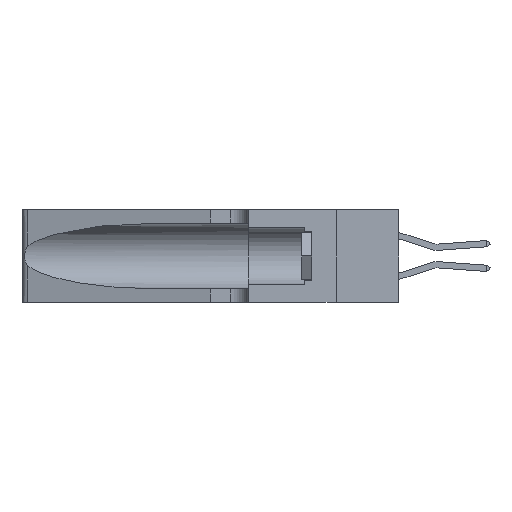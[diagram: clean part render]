
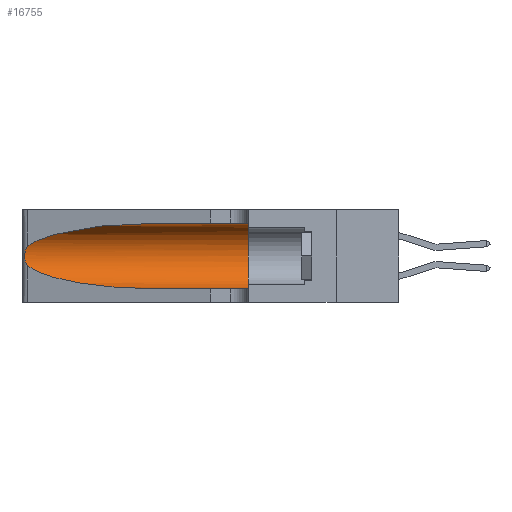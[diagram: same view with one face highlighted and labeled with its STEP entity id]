
A CAD part, left-side view. The second image highlights one B-rep face of the part: STEP entity #16755.
In plain terms, the highlighted cylindrical face has radius 3.308 mm (diameter 6.617 mm), a partial arc.
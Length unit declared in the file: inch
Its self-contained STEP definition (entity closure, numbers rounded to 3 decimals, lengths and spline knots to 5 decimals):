
#390 = VERTEX_POINT ( 'NONE', #656 ) ;
#656 = CARTESIAN_POINT ( 'NONE',  ( 0.1305, 0.35, 0.05475 ) ) ;
#829 = ORIENTED_EDGE ( 'NONE', *, *, #35304, .F. ) ;
#1144 = EDGE_CURVE ( 'NONE', #29607, #32186, #32940, .T. ) ;
#1484 = DIRECTION ( 'NONE',  ( 0., 0., -1. ) ) ;
#1635 = VERTEX_POINT ( 'NONE', #23614 ) ;
#3632 = CARTESIAN_POINT ( 'NONE',  ( 0.25555, 1.22993, 0.14849 ) ) ;
#4254 = CARTESIAN_POINT ( 'NONE',  ( 0.18966, 0.96281, 0.05475 ) ) ;
#4380 = CARTESIAN_POINT ( 'NONE',  ( 0.1305, 1.61858, 0.185 ) ) ;
#4558 = ORIENTED_EDGE ( 'NONE', *, *, #1144, .T. ) ;
#5376 = VECTOR ( 'NONE', #12789, 39.37008 ) ;
#6652 = EDGE_CURVE ( 'NONE', #27909, #29607, #11168, .T. ) ;
#6668 = ORIENTED_EDGE ( 'NONE', *, *, #27899, .T. ) ;
#6998 = CARTESIAN_POINT ( 'NONE',  ( 0.25789, 1.23486, 0.15765 ) ) ;
#7137 = CARTESIAN_POINT ( 'NONE',  ( 0.25555, 1.22994, 0.2215 ) ) ;
#7520 = FACE_OUTER_BOUND ( 'NONE', #35198, .T. ) ;
#7608 = CARTESIAN_POINT ( 'NONE',  ( 0.25487, 1.22718, 0.14631 ) ) ;
#8059 = EDGE_CURVE ( 'NONE', #1635, #27909, #25760, .T. ) ;
#9537 = CARTESIAN_POINT ( 'NONE',  ( 0.25487, 1.22718, 0.14631 ) ) ;
#10069 = CARTESIAN_POINT ( 'NONE',  ( 0.26018, 1.23835, 0.19895 ) ) ;
#11168 = B_SPLINE_CURVE_WITH_KNOTS ( 'NONE', 3,
 ( #29820, #7137, #30094, #43023, #23140, #10069, #26786, #39811, #36946, #39675, #6998, #33306, #3632, #30233 ),
 .UNSPECIFIED., .F., .F.,
 ( 4, 2, 2, 2, 2, 2, 4 ),
 ( 0., 0.00027, 0.00053, 0.00107, 0.0016, 0.00187, 0.00214 ),
 .UNSPECIFIED. ) ;
#11863 = CARTESIAN_POINT ( 'NONE',  ( 0.1305, 0.72297, 0.05475 ) ) ;
#12789 = DIRECTION ( 'NONE',  ( 0., -1., 0. ) ) ;
#14863 = CYLINDRICAL_SURFACE ( 'NONE', #21167, 0.13025 ) ;
#15998 = EDGE_CURVE ( 'NONE', #28734, #390, #23741, .T. ) ;
#16018 = CARTESIAN_POINT ( 'NONE',  ( 0.18966, 0.96281, 0.31525 ) ) ;
#16755 = ADVANCED_FACE ( 'NONE', ( #7520 ), #14863, .F. ) ;
#17876 = CARTESIAN_POINT ( 'NONE',  ( 0.1305, 0.35, 0.185 ) ) ;
#18676 = CARTESIAN_POINT ( 'NONE',  ( 0.1305, 1.61858, 0.05475 ) ) ;
#20584 = AXIS2_PLACEMENT_3D ( 'NONE', #17876, #34741, #35028 ) ;
#21167 = AXIS2_PLACEMENT_3D ( 'NONE', #4380, #34636, #1484 ) ;
#22700 = VECTOR ( 'NONE', #31290, 39.37008 ) ;
#23140 = CARTESIAN_POINT ( 'NONE',  ( 0.25854, 1.2359, 0.20912 ) ) ;
#23196 = CARTESIAN_POINT ( 'NONE',  ( 0.1305, 0.35, 0.31525 ) ) ;
#23614 = CARTESIAN_POINT ( 'NONE',  ( 0.1305, 0.72297, 0.31525 ) ) ;
#23741 = CIRCLE ( 'NONE', #20584, 0.13025 ) ;
#25760 =( BOUNDED_CURVE ( )  B_SPLINE_CURVE ( 3, ( #32696, #16018, #42717, #32416 ),
 .UNSPECIFIED., .F., .F. ) 
 B_SPLINE_CURVE_WITH_KNOTS ( ( 4, 4 ),
 ( 1.5708, 2.84003 ),
 .UNSPECIFIED. ) 
 CURVE ( )  GEOMETRIC_REPRESENTATION_ITEM ( )  RATIONAL_B_SPLINE_CURVE ( ( 1., 0.87, 0.87, 1. ) ) 
 REPRESENTATION_ITEM ( '' )  );
#26551 = ORIENTED_EDGE ( 'NONE', *, *, #6652, .T. ) ;
#26786 = CARTESIAN_POINT ( 'NONE',  ( 0.26075, 1.23896, 0.19203 ) ) ;
#27537 = CARTESIAN_POINT ( 'NONE',  ( 0.1305, 0.72297, 0.05475 ) ) ;
#27759 = ORIENTED_EDGE ( 'NONE', *, *, #15998, .F. ) ;
#27899 = EDGE_CURVE ( 'NONE', #32186, #390, #40351, .T. ) ;
#27909 = VERTEX_POINT ( 'NONE', #42315 ) ;
#28666 = ORIENTED_EDGE ( 'NONE', *, *, #8059, .T. ) ;
#28734 = VERTEX_POINT ( 'NONE', #23196 ) ;
#29607 = VERTEX_POINT ( 'NONE', #9537 ) ;
#29820 = CARTESIAN_POINT ( 'NONE',  ( 0.25487, 1.22718, 0.22369 ) ) ;
#30094 = CARTESIAN_POINT ( 'NONE',  ( 0.25639, 1.23184, 0.21858 ) ) ;
#30233 = CARTESIAN_POINT ( 'NONE',  ( 0.25487, 1.22718, 0.14631 ) ) ;
#31290 = DIRECTION ( 'NONE',  ( 0., -1., 0. ) ) ;
#32186 = VERTEX_POINT ( 'NONE', #11863 ) ;
#32416 = CARTESIAN_POINT ( 'NONE',  ( 0.25487, 1.22718, 0.22369 ) ) ;
#32696 = CARTESIAN_POINT ( 'NONE',  ( 0.1305, 0.72297, 0.31525 ) ) ;
#32940 =( BOUNDED_CURVE ( )  B_SPLINE_CURVE ( 3, ( #7608, #37422, #4254, #27537 ),
 .UNSPECIFIED., .F., .F. ) 
 B_SPLINE_CURVE_WITH_KNOTS ( ( 4, 4 ),
 ( 3.44316, 4.71239 ),
 .UNSPECIFIED. ) 
 CURVE ( )  GEOMETRIC_REPRESENTATION_ITEM ( )  RATIONAL_B_SPLINE_CURVE ( ( 1., 0.87, 0.87, 1. ) ) 
 REPRESENTATION_ITEM ( '' )  );
#33306 = CARTESIAN_POINT ( 'NONE',  ( 0.25639, 1.23186, 0.15144 ) ) ;
#34636 = DIRECTION ( 'NONE',  ( 0., -1., 0. ) ) ;
#34741 = DIRECTION ( 'NONE',  ( 0., 1., 0. ) ) ;
#35028 = DIRECTION ( 'NONE',  ( 0., 0., 1. ) ) ;
#35198 = EDGE_LOOP ( 'NONE', ( #28666, #26551, #4558, #6668, #27759, #829 ) ) ;
#35304 = EDGE_CURVE ( 'NONE', #1635, #28734, #38166, .T. ) ;
#36028 = CARTESIAN_POINT ( 'NONE',  ( 0.1305, 1.61858, 0.31525 ) ) ;
#36946 = CARTESIAN_POINT ( 'NONE',  ( 0.26017, 1.23833, 0.17102 ) ) ;
#37422 = CARTESIAN_POINT ( 'NONE',  ( 0.2373, 1.15595, 0.08982 ) ) ;
#38166 = LINE ( 'NONE', #36028, #5376 ) ;
#39675 = CARTESIAN_POINT ( 'NONE',  ( 0.25856, 1.23593, 0.16098 ) ) ;
#39811 = CARTESIAN_POINT ( 'NONE',  ( 0.26075, 1.23896, 0.178 ) ) ;
#40351 = LINE ( 'NONE', #18676, #22700 ) ;
#42315 = CARTESIAN_POINT ( 'NONE',  ( 0.25487, 1.22718, 0.22369 ) ) ;
#42717 = CARTESIAN_POINT ( 'NONE',  ( 0.2373, 1.15595, 0.28018 ) ) ;
#43023 = CARTESIAN_POINT ( 'NONE',  ( 0.25787, 1.23484, 0.2124 ) ) ;
